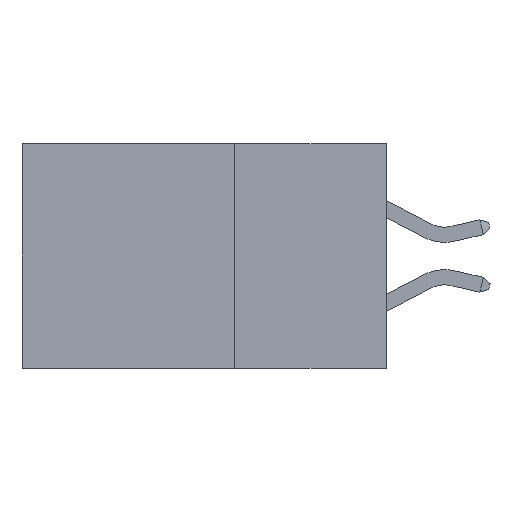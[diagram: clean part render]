
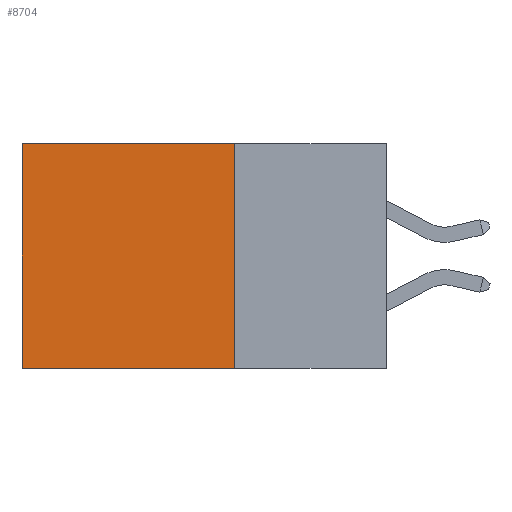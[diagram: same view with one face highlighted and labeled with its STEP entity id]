
A CAD part, left-side view. The second image highlights one B-rep face of the part: STEP entity #8704.
In plain terms, the highlighted planar face has unit normal (-1, 0, 0).
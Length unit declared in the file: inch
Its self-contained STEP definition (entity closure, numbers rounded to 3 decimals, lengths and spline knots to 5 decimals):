
#924 = ORIENTED_EDGE ( 'NONE', *, *, #8253, .T. ) ;
#1371 = EDGE_CURVE ( 'NONE', #11707, #16224, #16959, .T. ) ;
#3133 = EDGE_CURVE ( 'NONE', #16224, #10151, #3286, .T. ) ;
#3286 = LINE ( 'NONE', #9928, #4199 ) ;
#3670 = DIRECTION ( 'NONE',  ( 0., 0., -1. ) ) ;
#3873 = EDGE_CURVE ( 'NONE', #11707, #22871, #21462, .T. ) ;
#4151 = VECTOR ( 'NONE', #14336, 39.37008 ) ;
#4199 = VECTOR ( 'NONE', #17858, 39.37008 ) ;
#5768 = PLANE ( 'NONE',  #8322 ) ;
#8029 = VECTOR ( 'NONE', #9967, 39.37008 ) ;
#8253 = EDGE_CURVE ( 'NONE', #22871, #10151, #13246, .T. ) ;
#8289 = FACE_OUTER_BOUND ( 'NONE', #14208, .T. ) ;
#8322 = AXIS2_PLACEMENT_3D ( 'NONE', #23594, #13751, #21431 ) ;
#8704 = ADVANCED_FACE ( 'NONE', ( #8289 ), #5768, .F. ) ;
#9073 = ORIENTED_EDGE ( 'NONE', *, *, #1371, .F. ) ;
#9928 = CARTESIAN_POINT ( 'NONE',  ( 0.298, 0.25, -0.37 ) ) ;
#9967 = DIRECTION ( 'NONE',  ( 0., 0., -1. ) ) ;
#10151 = VERTEX_POINT ( 'NONE', #15784 ) ;
#10394 = CARTESIAN_POINT ( 'NONE',  ( 0.298, 0.25, 0. ) ) ;
#10617 = CARTESIAN_POINT ( 'NONE',  ( 0.298, 0.25, 0. ) ) ;
#11707 = VERTEX_POINT ( 'NONE', #10617 ) ;
#13246 = LINE ( 'NONE', #25463, #8029 ) ;
#13751 = DIRECTION ( 'NONE',  ( 1., 0., 0. ) ) ;
#14208 = EDGE_LOOP ( 'NONE', ( #924, #20860, #9073, #20476 ) ) ;
#14336 = DIRECTION ( 'NONE',  ( 0., 1., 0. ) ) ;
#15784 = CARTESIAN_POINT ( 'NONE',  ( 0.298, 0.6, -0.37 ) ) ;
#16224 = VERTEX_POINT ( 'NONE', #21951 ) ;
#16672 = CARTESIAN_POINT ( 'NONE',  ( 0.298, 0.6, 0. ) ) ;
#16959 = LINE ( 'NONE', #19201, #24132 ) ;
#17858 = DIRECTION ( 'NONE',  ( 0., 1., 0. ) ) ;
#19201 = CARTESIAN_POINT ( 'NONE',  ( 0.298, 0.25, 0. ) ) ;
#20476 = ORIENTED_EDGE ( 'NONE', *, *, #3873, .T. ) ;
#20860 = ORIENTED_EDGE ( 'NONE', *, *, #3133, .F. ) ;
#21431 = DIRECTION ( 'NONE',  ( 0., 0., -1. ) ) ;
#21462 = LINE ( 'NONE', #10394, #4151 ) ;
#21951 = CARTESIAN_POINT ( 'NONE',  ( 0.298, 0.25, -0.37 ) ) ;
#22871 = VERTEX_POINT ( 'NONE', #16672 ) ;
#23594 = CARTESIAN_POINT ( 'NONE',  ( 0.298, 0.25, 0. ) ) ;
#24132 = VECTOR ( 'NONE', #3670, 39.37008 ) ;
#25463 = CARTESIAN_POINT ( 'NONE',  ( 0.298, 0.6, 0. ) ) ;
